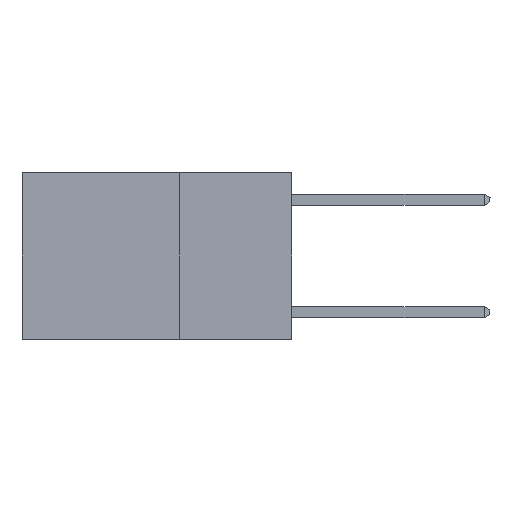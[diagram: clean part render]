
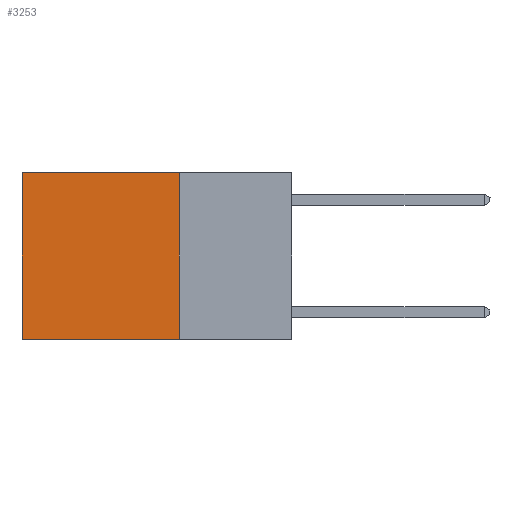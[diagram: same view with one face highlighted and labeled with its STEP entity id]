
A CAD part, left-side view. The second image highlights one B-rep face of the part: STEP entity #3253.
In plain terms, the highlighted planar face has unit normal (-1, 0, 0).
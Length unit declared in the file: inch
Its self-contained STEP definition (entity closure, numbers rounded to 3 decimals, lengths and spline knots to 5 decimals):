
#658 = CARTESIAN_POINT ( 'NONE',  ( 0.2625, 0.25, 0. ) ) ;
#678 = CARTESIAN_POINT ( 'NONE',  ( 0.2625, 0.25, 0. ) ) ;
#701 = VERTEX_POINT ( 'NONE', #1899 ) ;
#1163 = VECTOR ( 'NONE', #2212, 39.37008 ) ;
#1328 = LINE ( 'NONE', #9411, #9791 ) ;
#1899 = CARTESIAN_POINT ( 'NONE',  ( 0.2625, 0.25, -0.37 ) ) ;
#2212 = DIRECTION ( 'NONE',  ( 0., 1., 0. ) ) ;
#2337 = ORIENTED_EDGE ( 'NONE', *, *, #8788, .F. ) ;
#3208 = VECTOR ( 'NONE', #12731, 39.37008 ) ;
#3253 = ADVANCED_FACE ( 'NONE', ( #10623 ), #12246, .F. ) ;
#3612 = CARTESIAN_POINT ( 'NONE',  ( 0.2625, 0.25, 0. ) ) ;
#3891 = LINE ( 'NONE', #11704, #3208 ) ;
#4070 = LINE ( 'NONE', #8551, #1163 ) ;
#4187 = ORIENTED_EDGE ( 'NONE', *, *, #7570, .F. ) ;
#4519 = ORIENTED_EDGE ( 'NONE', *, *, #4764, .T. ) ;
#4547 = AXIS2_PLACEMENT_3D ( 'NONE', #658, #6109, #13275 ) ;
#4745 = VERTEX_POINT ( 'NONE', #9378 ) ;
#4764 = EDGE_CURVE ( 'NONE', #11154, #4745, #4070, .T. ) ;
#6109 = DIRECTION ( 'NONE',  ( 1., 0., 0. ) ) ;
#7570 = EDGE_CURVE ( 'NONE', #701, #13463, #3891, .T. ) ;
#7743 = EDGE_LOOP ( 'NONE', ( #11605, #4187, #2337, #4519 ) ) ;
#8551 = CARTESIAN_POINT ( 'NONE',  ( 0.2625, 0.25, 0. ) ) ;
#8788 = EDGE_CURVE ( 'NONE', #11154, #701, #12433, .T. ) ;
#9378 = CARTESIAN_POINT ( 'NONE',  ( 0.2625, 0.6, 0. ) ) ;
#9411 = CARTESIAN_POINT ( 'NONE',  ( 0.2625, 0.6, 0. ) ) ;
#9740 = VECTOR ( 'NONE', #10246, 39.37008 ) ;
#9791 = VECTOR ( 'NONE', #11411, 39.37008 ) ;
#10246 = DIRECTION ( 'NONE',  ( 0., 0., -1. ) ) ;
#10623 = FACE_OUTER_BOUND ( 'NONE', #7743, .T. ) ;
#11154 = VERTEX_POINT ( 'NONE', #3612 ) ;
#11265 = CARTESIAN_POINT ( 'NONE',  ( 0.2625, 0.6, -0.37 ) ) ;
#11411 = DIRECTION ( 'NONE',  ( 0., 0., -1. ) ) ;
#11605 = ORIENTED_EDGE ( 'NONE', *, *, #13120, .T. ) ;
#11704 = CARTESIAN_POINT ( 'NONE',  ( 0.2625, 0.25, -0.37 ) ) ;
#12246 = PLANE ( 'NONE',  #4547 ) ;
#12433 = LINE ( 'NONE', #678, #9740 ) ;
#12731 = DIRECTION ( 'NONE',  ( 0., 1., 0. ) ) ;
#13120 = EDGE_CURVE ( 'NONE', #4745, #13463, #1328, .T. ) ;
#13275 = DIRECTION ( 'NONE',  ( 0., 0., -1. ) ) ;
#13463 = VERTEX_POINT ( 'NONE', #11265 ) ;
